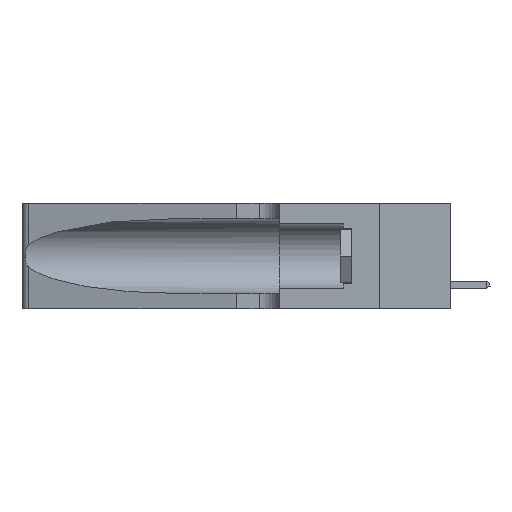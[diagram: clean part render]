
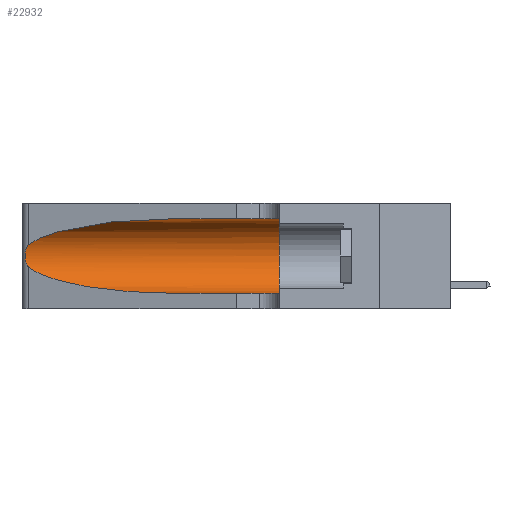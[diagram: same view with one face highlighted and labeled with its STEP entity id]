
A CAD part, left-side view. The second image highlights one B-rep face of the part: STEP entity #22932.
In plain terms, the highlighted cylindrical face has radius 3.308 mm (diameter 6.617 mm), a partial arc.
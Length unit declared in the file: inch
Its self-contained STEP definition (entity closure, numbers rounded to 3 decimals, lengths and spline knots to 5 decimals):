
#34 = ORIENTED_EDGE ( 'NONE', *, *, #211, .F. ) ;
#211 = EDGE_CURVE ( 'NONE', #5705, #17122, #9060, .T. ) ;
#978 = CARTESIAN_POINT ( 'NONE',  ( 0.25487, 1.22718, 0.22369 ) ) ;
#1057 = CARTESIAN_POINT ( 'NONE',  ( 0.25787, 1.23484, 0.2124 ) ) ;
#1095 = B_SPLINE_CURVE_WITH_KNOTS ( 'NONE', 3,
 ( #978, #15244, #19096, #1057, #13601, #8327, #8091, #22652, #1137, #13452, #13666, #15466, #6564, #6403 ),
 .UNSPECIFIED., .F., .F.,
 ( 4, 2, 2, 2, 2, 2, 4 ),
 ( 0., 0.00027, 0.00053, 0.00107, 0.0016, 0.00187, 0.00214 ),
 .UNSPECIFIED. ) ;
#1137 = CARTESIAN_POINT ( 'NONE',  ( 0.26017, 1.23833, 0.17102 ) ) ;
#1475 = CARTESIAN_POINT ( 'NONE',  ( 0.2373, 1.15595, 0.08982 ) ) ;
#2055 = CARTESIAN_POINT ( 'NONE',  ( 0.2373, 1.15595, 0.28018 ) ) ;
#3012 = CYLINDRICAL_SURFACE ( 'NONE', #11547, 0.13025 ) ;
#3210 = CARTESIAN_POINT ( 'NONE',  ( 0.25487, 1.22718, 0.14631 ) ) ;
#3249 = DIRECTION ( 'NONE',  ( 0., 1., 0. ) ) ;
#3797 = CARTESIAN_POINT ( 'NONE',  ( 0.1305, 1.61858, 0.31525 ) ) ;
#4136 = DIRECTION ( 'NONE',  ( 0., -1., 0. ) ) ;
#4908 = DIRECTION ( 'NONE',  ( 0., 0., 1. ) ) ;
#4911 = VECTOR ( 'NONE', #4136, 39.37008 ) ;
#5578 = ORIENTED_EDGE ( 'NONE', *, *, #9555, .T. ) ;
#5705 = VERTEX_POINT ( 'NONE', #21049 ) ;
#5729 = EDGE_CURVE ( 'NONE', #17122, #9432, #19716, .T. ) ;
#5859 = CARTESIAN_POINT ( 'NONE',  ( 0.1305, 1.61858, 0.05475 ) ) ;
#6403 = CARTESIAN_POINT ( 'NONE',  ( 0.25487, 1.22718, 0.14631 ) ) ;
#6564 = CARTESIAN_POINT ( 'NONE',  ( 0.25555, 1.22993, 0.14849 ) ) ;
#7656 = CARTESIAN_POINT ( 'NONE',  ( 0.1305, 1.61858, 0.185 ) ) ;
#8091 = CARTESIAN_POINT ( 'NONE',  ( 0.26075, 1.23896, 0.19203 ) ) ;
#8327 = CARTESIAN_POINT ( 'NONE',  ( 0.26018, 1.23835, 0.19895 ) ) ;
#8876 = ORIENTED_EDGE ( 'NONE', *, *, #5729, .F. ) ;
#8954 = FACE_OUTER_BOUND ( 'NONE', #19658, .T. ) ;
#9060 = LINE ( 'NONE', #3797, #17727 ) ;
#9231 = DIRECTION ( 'NONE',  ( 0., 0., -1. ) ) ;
#9304 = DIRECTION ( 'NONE',  ( 0., -1., 0. ) ) ;
#9432 = VERTEX_POINT ( 'NONE', #17999 ) ;
#9484 =( BOUNDED_CURVE ( )  B_SPLINE_CURVE ( 3, ( #21450, #12709, #2055, #18125 ),
 .UNSPECIFIED., .F., .T. ) 
 B_SPLINE_CURVE_WITH_KNOTS ( ( 4, 4 ),
 ( 1.5708, 2.84003 ),
 .UNSPECIFIED. ) 
 CURVE ( )  GEOMETRIC_REPRESENTATION_ITEM ( )  RATIONAL_B_SPLINE_CURVE ( ( 1., 0.87, 0.87, 1. ) ) 
 REPRESENTATION_ITEM ( '' )  );
#9555 = EDGE_CURVE ( 'NONE', #14668, #9432, #16419, .T. ) ;
#11500 = ORIENTED_EDGE ( 'NONE', *, *, #22216, .T. ) ;
#11547 = AXIS2_PLACEMENT_3D ( 'NONE', #7656, #9304, #9231 ) ;
#12020 = CARTESIAN_POINT ( 'NONE',  ( 0.1305, 0.35, 0.185 ) ) ;
#12463 = VERTEX_POINT ( 'NONE', #16340 ) ;
#12612 = CARTESIAN_POINT ( 'NONE',  ( 0.1305, 0.35, 0.31525 ) ) ;
#12709 = CARTESIAN_POINT ( 'NONE',  ( 0.18966, 0.96281, 0.31525 ) ) ;
#13452 = CARTESIAN_POINT ( 'NONE',  ( 0.25856, 1.23593, 0.16098 ) ) ;
#13601 = CARTESIAN_POINT ( 'NONE',  ( 0.25854, 1.2359, 0.20912 ) ) ;
#13614 = ORIENTED_EDGE ( 'NONE', *, *, #17080, .T. ) ;
#13666 = CARTESIAN_POINT ( 'NONE',  ( 0.25789, 1.23486, 0.15765 ) ) ;
#13998 = CARTESIAN_POINT ( 'NONE',  ( 0.1305, 0.72297, 0.05475 ) ) ;
#14282 = DIRECTION ( 'NONE',  ( 0., -1., 0. ) ) ;
#14668 = VERTEX_POINT ( 'NONE', #13998 ) ;
#15244 = CARTESIAN_POINT ( 'NONE',  ( 0.25555, 1.22994, 0.2215 ) ) ;
#15466 = CARTESIAN_POINT ( 'NONE',  ( 0.25639, 1.23186, 0.15144 ) ) ;
#15820 = CARTESIAN_POINT ( 'NONE',  ( 0.1305, 0.72297, 0.05475 ) ) ;
#15907 = CARTESIAN_POINT ( 'NONE',  ( 0.18966, 0.96281, 0.05475 ) ) ;
#16340 = CARTESIAN_POINT ( 'NONE',  ( 0.25487, 1.22718, 0.14631 ) ) ;
#16419 = LINE ( 'NONE', #5859, #4911 ) ;
#17080 = EDGE_CURVE ( 'NONE', #12463, #14668, #21990, .T. ) ;
#17122 = VERTEX_POINT ( 'NONE', #12612 ) ;
#17616 = AXIS2_PLACEMENT_3D ( 'NONE', #12020, #3249, #4908 ) ;
#17727 = VECTOR ( 'NONE', #14282, 39.37008 ) ;
#17999 = CARTESIAN_POINT ( 'NONE',  ( 0.1305, 0.35, 0.05475 ) ) ;
#18125 = CARTESIAN_POINT ( 'NONE',  ( 0.25487, 1.22718, 0.22369 ) ) ;
#19095 = EDGE_CURVE ( 'NONE', #5705, #21778, #9484, .T. ) ;
#19096 = CARTESIAN_POINT ( 'NONE',  ( 0.25639, 1.23184, 0.21858 ) ) ;
#19658 = EDGE_LOOP ( 'NONE', ( #20935, #11500, #13614, #5578, #8876, #34 ) ) ;
#19716 = CIRCLE ( 'NONE', #17616, 0.13025 ) ;
#20882 = CARTESIAN_POINT ( 'NONE',  ( 0.25487, 1.22718, 0.22369 ) ) ;
#20935 = ORIENTED_EDGE ( 'NONE', *, *, #19095, .T. ) ;
#21049 = CARTESIAN_POINT ( 'NONE',  ( 0.1305, 0.72297, 0.31525 ) ) ;
#21450 = CARTESIAN_POINT ( 'NONE',  ( 0.1305, 0.72297, 0.31525 ) ) ;
#21778 = VERTEX_POINT ( 'NONE', #20882 ) ;
#21990 =( BOUNDED_CURVE ( )  B_SPLINE_CURVE ( 3, ( #3210, #1475, #15907, #15820 ),
 .UNSPECIFIED., .F., .F. ) 
 B_SPLINE_CURVE_WITH_KNOTS ( ( 4, 4 ),
 ( 3.44316, 4.71239 ),
 .UNSPECIFIED. ) 
 CURVE ( )  GEOMETRIC_REPRESENTATION_ITEM ( )  RATIONAL_B_SPLINE_CURVE ( ( 1., 0.87, 0.87, 1. ) ) 
 REPRESENTATION_ITEM ( '' )  );
#22216 = EDGE_CURVE ( 'NONE', #21778, #12463, #1095, .T. ) ;
#22652 = CARTESIAN_POINT ( 'NONE',  ( 0.26075, 1.23896, 0.178 ) ) ;
#22932 = ADVANCED_FACE ( 'NONE', ( #8954 ), #3012, .F. ) ;
